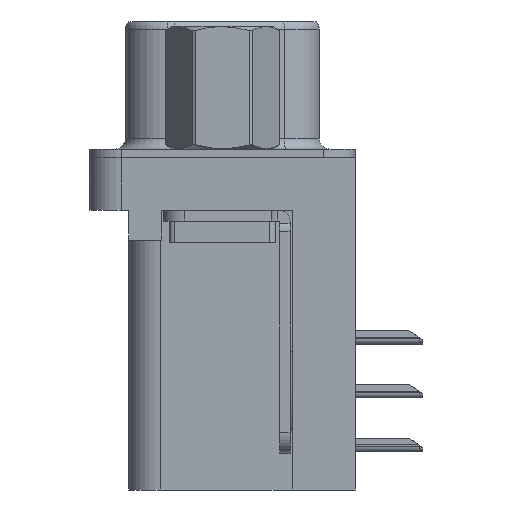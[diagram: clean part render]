
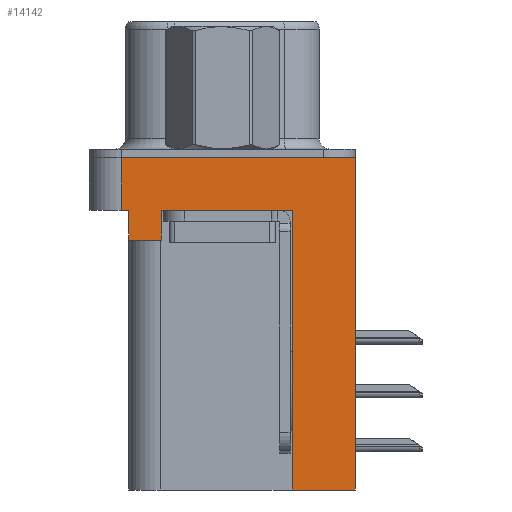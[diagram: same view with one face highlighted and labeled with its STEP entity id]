
A CAD part, left-side view. The second image highlights one B-rep face of the part: STEP entity #14142.
In plain terms, the highlighted planar face has unit normal (-1, 0, 0).
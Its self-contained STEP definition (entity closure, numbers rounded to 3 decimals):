
#488 = VERTEX_POINT ( 'NONE', #34279 ) ;
#1059 = CARTESIAN_POINT ( 'NONE',  ( -3., 4.425, -2.5 ) ) ;
#1482 = EDGE_CURVE ( 'NONE', #9690, #7270, #30083, .T. ) ;
#1646 = CARTESIAN_POINT ( 'NONE',  ( -3., 4.775, -2.5 ) ) ;
#1752 = DIRECTION ( 'NONE',  ( 0., -1., 0. ) ) ;
#2563 = DIRECTION ( 'NONE',  ( 0., 1., 0. ) ) ;
#2757 = DIRECTION ( 'NONE',  ( 0., 0., 1. ) ) ;
#3452 = VECTOR ( 'NONE', #15677, 1000. ) ;
#5477 = EDGE_CURVE ( 'NONE', #14215, #7270, #11299, .T. ) ;
#6874 = VECTOR ( 'NONE', #14588, 1000. ) ;
#7270 = VERTEX_POINT ( 'NONE', #27952 ) ;
#7383 = CARTESIAN_POINT ( 'NONE',  ( -3., -6.275, -15.7 ) ) ;
#7627 = VERTEX_POINT ( 'NONE', #7383 ) ;
#7807 = DIRECTION ( 'NONE',  ( 0., 0., 1. ) ) ;
#7939 = DIRECTION ( 'NONE',  ( 0., -1., 0. ) ) ;
#9299 = ORIENTED_EDGE ( 'NONE', *, *, #20926, .T. ) ;
#9452 = DIRECTION ( 'NONE',  ( 0., 0., 1. ) ) ;
#9690 = VERTEX_POINT ( 'NONE', #21160 ) ;
#10343 = EDGE_CURVE ( 'NONE', #34808, #31842, #20120, .T. ) ;
#10391 = CARTESIAN_POINT ( 'NONE',  ( -3., 4.775, -2.5 ) ) ;
#10510 = EDGE_LOOP ( 'NONE', ( #24414, #32794, #35472, #12499, #15657, #19305, #17219, #32212, #18993, #9299 ) ) ;
#11087 = DIRECTION ( 'NONE',  ( 0., 0., 1. ) ) ;
#11096 = VECTOR ( 'NONE', #7939, 1000. ) ;
#11299 = LINE ( 'NONE', #25879, #25891 ) ;
#11939 = LINE ( 'NONE', #25686, #16671 ) ;
#12161 = FACE_OUTER_BOUND ( 'NONE', #10510, .T. ) ;
#12191 = CARTESIAN_POINT ( 'NONE',  ( -3., -3.295, -15.7 ) ) ;
#12499 = ORIENTED_EDGE ( 'NONE', *, *, #34970, .F. ) ;
#12746 = VECTOR ( 'NONE', #7807, 1000. ) ;
#12942 = VECTOR ( 'NONE', #25899, 1000. ) ;
#14142 = ADVANCED_FACE ( 'NONE', ( #12161 ), #19264, .T. ) ;
#14215 = VERTEX_POINT ( 'NONE', #16716 ) ;
#14588 = DIRECTION ( 'NONE',  ( 0., -1., 0. ) ) ;
#15657 = ORIENTED_EDGE ( 'NONE', *, *, #26905, .F. ) ;
#15677 = DIRECTION ( 'NONE',  ( 0., 0., 1. ) ) ;
#16671 = VECTOR ( 'NONE', #20196, 1000. ) ;
#16716 = CARTESIAN_POINT ( 'NONE',  ( -3., -3.295, -15.7 ) ) ;
#17219 = ORIENTED_EDGE ( 'NONE', *, *, #1482, .T. ) ;
#17780 = AXIS2_PLACEMENT_3D ( 'NONE', #22043, #27511, #11087 ) ;
#18163 = VECTOR ( 'NONE', #2563, 1000. ) ;
#18211 = EDGE_CURVE ( 'NONE', #34808, #20069, #33879, .T. ) ;
#18616 = CARTESIAN_POINT ( 'NONE',  ( -3., 2.895, -3.9 ) ) ;
#18782 = VERTEX_POINT ( 'NONE', #18616 ) ;
#18993 = ORIENTED_EDGE ( 'NONE', *, *, #30144, .F. ) ;
#19036 = LINE ( 'NONE', #21851, #18163 ) ;
#19264 = PLANE ( 'NONE',  #17780 ) ;
#19305 = ORIENTED_EDGE ( 'NONE', *, *, #33896, .T. ) ;
#19999 = CARTESIAN_POINT ( 'NONE',  ( -3., -6.275, -2.5 ) ) ;
#20069 = VERTEX_POINT ( 'NONE', #1059 ) ;
#20120 = LINE ( 'NONE', #1646, #12746 ) ;
#20196 = DIRECTION ( 'NONE',  ( 0., 0., 1. ) ) ;
#20736 = CARTESIAN_POINT ( 'NONE',  ( -3., -6.275, 0. ) ) ;
#20926 = EDGE_CURVE ( 'NONE', #7627, #27282, #25405, .T. ) ;
#21160 = CARTESIAN_POINT ( 'NONE',  ( -3., 2.895, -2.5 ) ) ;
#21169 = LINE ( 'NONE', #12191, #12942 ) ;
#21393 = EDGE_CURVE ( 'NONE', #31842, #27282, #21520, .T. ) ;
#21520 = LINE ( 'NONE', #33851, #6874 ) ;
#21851 = CARTESIAN_POINT ( 'NONE',  ( -3., 4.425, -3.9 ) ) ;
#22043 = CARTESIAN_POINT ( 'NONE',  ( -3., -6.275, -2.5 ) ) ;
#22723 = CARTESIAN_POINT ( 'NONE',  ( -3., 4.775, 0. ) ) ;
#22784 = VECTOR ( 'NONE', #1752, 1000. ) ;
#24414 = ORIENTED_EDGE ( 'NONE', *, *, #21393, .F. ) ;
#25405 = LINE ( 'NONE', #29429, #3452 ) ;
#25639 = VECTOR ( 'NONE', #2757, 1000. ) ;
#25686 = CARTESIAN_POINT ( 'NONE',  ( -3., 2.895, -3.9 ) ) ;
#25879 = CARTESIAN_POINT ( 'NONE',  ( -3., -3.295, -15.7 ) ) ;
#25891 = VECTOR ( 'NONE', #9452, 1000. ) ;
#25899 = DIRECTION ( 'NONE',  ( 0., 1., 0. ) ) ;
#26905 = EDGE_CURVE ( 'NONE', #18782, #488, #19036, .T. ) ;
#27282 = VERTEX_POINT ( 'NONE', #20736 ) ;
#27511 = DIRECTION ( 'NONE',  ( -1., 0., 0. ) ) ;
#27952 = CARTESIAN_POINT ( 'NONE',  ( -3., -3.295, -2.5 ) ) ;
#29429 = CARTESIAN_POINT ( 'NONE',  ( -3., -6.275, -2.5 ) ) ;
#30083 = LINE ( 'NONE', #19999, #22784 ) ;
#30144 = EDGE_CURVE ( 'NONE', #7627, #14215, #21169, .T. ) ;
#31842 = VERTEX_POINT ( 'NONE', #22723 ) ;
#32212 = ORIENTED_EDGE ( 'NONE', *, *, #5477, .F. ) ;
#32705 = CARTESIAN_POINT ( 'NONE',  ( -3., -6.275, -2.5 ) ) ;
#32794 = ORIENTED_EDGE ( 'NONE', *, *, #10343, .F. ) ;
#33824 = LINE ( 'NONE', #34125, #25639 ) ;
#33851 = CARTESIAN_POINT ( 'NONE',  ( -3., -6.275, 0. ) ) ;
#33879 = LINE ( 'NONE', #32705, #11096 ) ;
#33896 = EDGE_CURVE ( 'NONE', #18782, #9690, #11939, .T. ) ;
#34125 = CARTESIAN_POINT ( 'NONE',  ( -3., 4.425, -3.9 ) ) ;
#34279 = CARTESIAN_POINT ( 'NONE',  ( -3., 4.425, -3.9 ) ) ;
#34808 = VERTEX_POINT ( 'NONE', #10391 ) ;
#34970 = EDGE_CURVE ( 'NONE', #488, #20069, #33824, .T. ) ;
#35472 = ORIENTED_EDGE ( 'NONE', *, *, #18211, .T. ) ;
